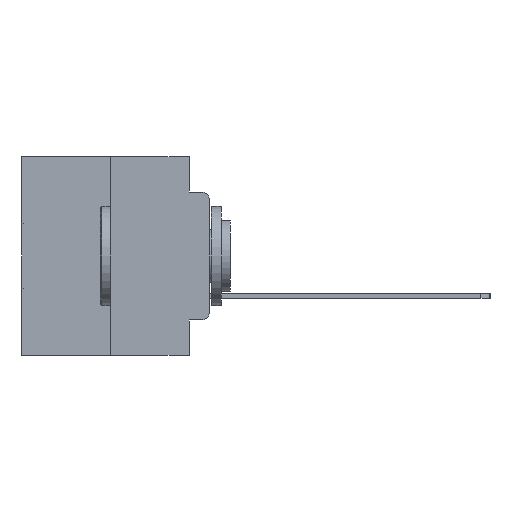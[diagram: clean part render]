
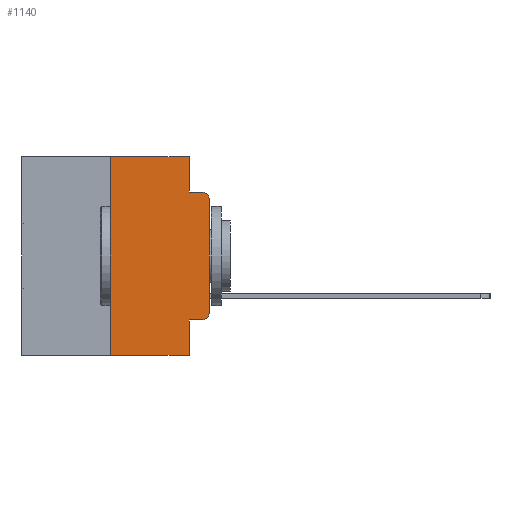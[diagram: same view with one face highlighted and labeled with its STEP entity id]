
A CAD part, left-side view. The second image highlights one B-rep face of the part: STEP entity #1140.
In plain terms, the highlighted planar face has unit normal (-1, 0, 0).
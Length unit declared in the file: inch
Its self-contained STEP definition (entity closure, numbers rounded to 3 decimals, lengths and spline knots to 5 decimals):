
#421 = VERTEX_POINT ( 'NONE', #14289 ) ;
#423 = ORIENTED_EDGE ( 'NONE', *, *, #1808, .F. ) ;
#451 = FACE_OUTER_BOUND ( 'NONE', #13037, .T. ) ;
#557 = LINE ( 'NONE', #14656, #29584 ) ;
#602 = DIRECTION ( 'NONE',  ( 0., -1., 0. ) ) ;
#1140 = ADVANCED_FACE ( 'NONE', ( #451 ), #5326, .F. ) ;
#1465 = DIRECTION ( 'NONE',  ( 0., 0., -1. ) ) ;
#1556 = LINE ( 'NONE', #17118, #19307 ) ;
#1808 = EDGE_CURVE ( 'NONE', #6982, #10782, #1556, .T. ) ;
#2469 = CARTESIAN_POINT ( 'NONE',  ( 0., 0.02, -0.0885 ) ) ;
#2544 = CARTESIAN_POINT ( 'NONE',  ( 0., 0.051, -0.4115 ) ) ;
#4088 = CARTESIAN_POINT ( 'NONE',  ( 0., 0.051, -0.4115 ) ) ;
#4915 = LINE ( 'NONE', #22741, #27824 ) ;
#4984 = EDGE_CURVE ( 'NONE', #10782, #23970, #29284, .T. ) ;
#5326 = PLANE ( 'NONE',  #9343 ) ;
#6251 = ORIENTED_EDGE ( 'NONE', *, *, #18031, .F. ) ;
#6625 = CARTESIAN_POINT ( 'NONE',  ( 0., 0.25, 0. ) ) ;
#6982 = VERTEX_POINT ( 'NONE', #9533 ) ;
#7396 = EDGE_CURVE ( 'NONE', #12053, #11311, #29184, .T. ) ;
#8803 = DIRECTION ( 'NONE',  ( 0., -1., 0. ) ) ;
#9101 = VERTEX_POINT ( 'NONE', #2469 ) ;
#9151 = DIRECTION ( 'NONE',  ( -1., 0., 0. ) ) ;
#9322 = AXIS2_PLACEMENT_3D ( 'NONE', #22962, #9151, #25232 ) ;
#9343 = AXIS2_PLACEMENT_3D ( 'NONE', #17656, #9435, #21479 ) ;
#9435 = DIRECTION ( 'NONE',  ( 1., 0., 0. ) ) ;
#9533 = CARTESIAN_POINT ( 'NONE',  ( 0., 0.25, -0.5 ) ) ;
#9802 = ORIENTED_EDGE ( 'NONE', *, *, #19070, .T. ) ;
#9966 = AXIS2_PLACEMENT_3D ( 'NONE', #28870, #15384, #1465 ) ;
#10086 = EDGE_CURVE ( 'NONE', #21186, #9101, #26199, .T. ) ;
#10101 = DIRECTION ( 'NONE',  ( 0., 0., 1. ) ) ;
#10782 = VERTEX_POINT ( 'NONE', #6625 ) ;
#11051 = VECTOR ( 'NONE', #8803, 39.37008 ) ;
#11171 = VECTOR ( 'NONE', #602, 39.37008 ) ;
#11311 = VERTEX_POINT ( 'NONE', #16164 ) ;
#12053 = VERTEX_POINT ( 'NONE', #2544 ) ;
#12670 = DIRECTION ( 'NONE',  ( 0., 0., -1. ) ) ;
#13037 = EDGE_LOOP ( 'NONE', ( #9802, #24209, #14984, #6251, #20727, #423, #27050, #15403, #21115, #22522 ) ) ;
#13077 = DIRECTION ( 'NONE',  ( 0., -1., 0. ) ) ;
#14289 = CARTESIAN_POINT ( 'NONE',  ( 0., 0., -0.3915 ) ) ;
#14656 = CARTESIAN_POINT ( 'NONE',  ( 0., 0., 0. ) ) ;
#14984 = ORIENTED_EDGE ( 'NONE', *, *, #10086, .F. ) ;
#15217 = VECTOR ( 'NONE', #12670, 39.37008 ) ;
#15384 = DIRECTION ( 'NONE',  ( -1., 0., 0. ) ) ;
#15403 = ORIENTED_EDGE ( 'NONE', *, *, #20474, .F. ) ;
#16022 = CIRCLE ( 'NONE', #9966, 0.02 ) ;
#16164 = CARTESIAN_POINT ( 'NONE',  ( 0., 0.02, -0.4115 ) ) ;
#16537 = CARTESIAN_POINT ( 'NONE',  ( 0., 0., -0.1085 ) ) ;
#17118 = CARTESIAN_POINT ( 'NONE',  ( 0., 0.25, 0. ) ) ;
#17656 = CARTESIAN_POINT ( 'NONE',  ( 0., 0.473, 0. ) ) ;
#18031 = EDGE_CURVE ( 'NONE', #23970, #21186, #27924, .T. ) ;
#18033 = CARTESIAN_POINT ( 'NONE',  ( 0., 0.051, -0.5 ) ) ;
#18759 = VERTEX_POINT ( 'NONE', #18033 ) ;
#19070 = EDGE_CURVE ( 'NONE', #421, #28690, #557, .T. ) ;
#19307 = VECTOR ( 'NONE', #10101, 39.37008 ) ;
#19882 = CARTESIAN_POINT ( 'NONE',  ( 0., 0.051, 0. ) ) ;
#20474 = EDGE_CURVE ( 'NONE', #12053, #18759, #4915, .T. ) ;
#20479 = VECTOR ( 'NONE', #20774, 39.37008 ) ;
#20542 = EDGE_CURVE ( 'NONE', #6982, #18759, #26430, .T. ) ;
#20688 = CIRCLE ( 'NONE', #9322, 0.02 ) ;
#20727 = ORIENTED_EDGE ( 'NONE', *, *, #4984, .F. ) ;
#20774 = DIRECTION ( 'NONE',  ( 0., -1., 0. ) ) ;
#21115 = ORIENTED_EDGE ( 'NONE', *, *, #7396, .T. ) ;
#21186 = VERTEX_POINT ( 'NONE', #25352 ) ;
#21479 = DIRECTION ( 'NONE',  ( 0., 0., -1. ) ) ;
#22175 = CARTESIAN_POINT ( 'NONE',  ( 0., 0.051, -0.0885 ) ) ;
#22522 = ORIENTED_EDGE ( 'NONE', *, *, #28376, .T. ) ;
#22741 = CARTESIAN_POINT ( 'NONE',  ( 0., 0.051, 0. ) ) ;
#22931 = EDGE_CURVE ( 'NONE', #28690, #9101, #20688, .T. ) ;
#22962 = CARTESIAN_POINT ( 'NONE',  ( 0., 0.02, -0.1085 ) ) ;
#23970 = VERTEX_POINT ( 'NONE', #19882 ) ;
#24209 = ORIENTED_EDGE ( 'NONE', *, *, #22931, .T. ) ;
#25195 = CARTESIAN_POINT ( 'NONE',  ( 0., 0.473, -0.5 ) ) ;
#25232 = DIRECTION ( 'NONE',  ( 0., 0., -1. ) ) ;
#25352 = CARTESIAN_POINT ( 'NONE',  ( 0., 0.051, -0.0885 ) ) ;
#25510 = VECTOR ( 'NONE', #13077, 39.37008 ) ;
#26199 = LINE ( 'NONE', #22175, #25510 ) ;
#26430 = LINE ( 'NONE', #25195, #20479 ) ;
#27050 = ORIENTED_EDGE ( 'NONE', *, *, #20542, .T. ) ;
#27246 = DIRECTION ( 'NONE',  ( 0., 0., -1. ) ) ;
#27824 = VECTOR ( 'NONE', #27246, 39.37008 ) ;
#27924 = LINE ( 'NONE', #28534, #15217 ) ;
#28084 = CARTESIAN_POINT ( 'NONE',  ( 0., 0.473, 0. ) ) ;
#28088 = DIRECTION ( 'NONE',  ( 0., 0., 1. ) ) ;
#28376 = EDGE_CURVE ( 'NONE', #11311, #421, #16022, .T. ) ;
#28534 = CARTESIAN_POINT ( 'NONE',  ( 0., 0.051, 0. ) ) ;
#28690 = VERTEX_POINT ( 'NONE', #16537 ) ;
#28870 = CARTESIAN_POINT ( 'NONE',  ( 0., 0.02, -0.3915 ) ) ;
#29184 = LINE ( 'NONE', #4088, #11051 ) ;
#29284 = LINE ( 'NONE', #28084, #11171 ) ;
#29584 = VECTOR ( 'NONE', #28088, 39.37008 ) ;
